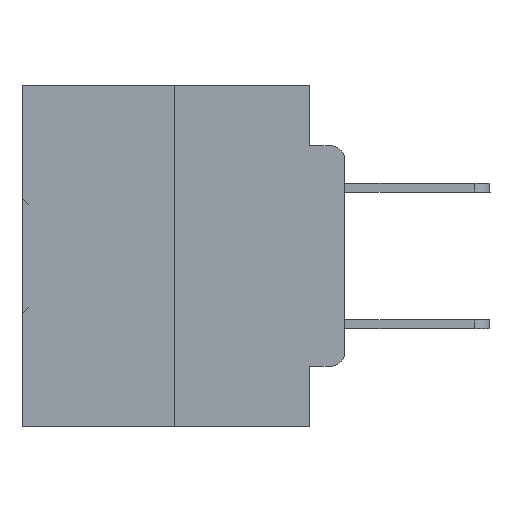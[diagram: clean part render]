
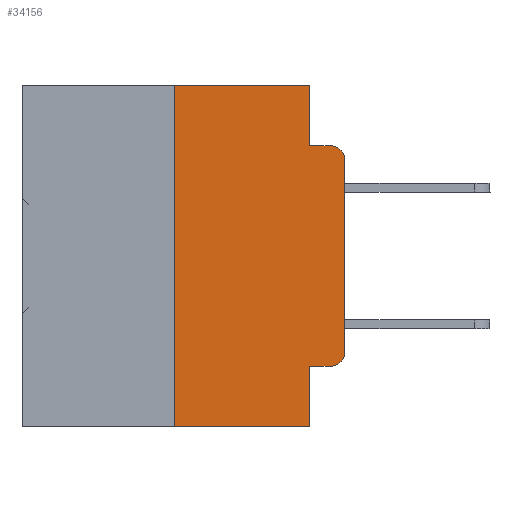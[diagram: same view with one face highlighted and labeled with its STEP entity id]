
A CAD part, left-side view. The second image highlights one B-rep face of the part: STEP entity #34156.
In plain terms, the highlighted planar face has unit normal (-1, 0, 0).
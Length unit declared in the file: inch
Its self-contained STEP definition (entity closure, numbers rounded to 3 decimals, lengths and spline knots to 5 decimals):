
#143 = VECTOR ( 'NONE', #10157, 39.37008 ) ;
#616 = ORIENTED_EDGE ( 'NONE', *, *, #23244, .F. ) ;
#656 = VERTEX_POINT ( 'NONE', #26328 ) ;
#908 = DIRECTION ( 'NONE',  ( -1., 0., 0. ) ) ;
#1549 = VERTEX_POINT ( 'NONE', #1915 ) ;
#1915 = CARTESIAN_POINT ( 'NONE',  ( 0., 0.051, -0.5 ) ) ;
#2710 = CARTESIAN_POINT ( 'NONE',  ( 0., 0.051, 0. ) ) ;
#4378 = EDGE_CURVE ( 'NONE', #37192, #1549, #31212, .T. ) ;
#4537 = VERTEX_POINT ( 'NONE', #11306 ) ;
#4974 = LINE ( 'NONE', #16615, #14057 ) ;
#5849 = CARTESIAN_POINT ( 'NONE',  ( 0., 0., 0. ) ) ;
#6620 = VECTOR ( 'NONE', #20495, 39.37008 ) ;
#6967 = EDGE_CURVE ( 'NONE', #656, #1549, #36945, .T. ) ;
#6978 = DIRECTION ( 'NONE',  ( 1., 0., 0. ) ) ;
#7118 = LINE ( 'NONE', #27726, #143 ) ;
#7808 = ORIENTED_EDGE ( 'NONE', *, *, #36953, .F. ) ;
#8787 = CARTESIAN_POINT ( 'NONE',  ( 0., 0.02, -0.0885 ) ) ;
#8930 = LINE ( 'NONE', #28993, #17694 ) ;
#9353 = AXIS2_PLACEMENT_3D ( 'NONE', #15770, #908, #24173 ) ;
#10157 = DIRECTION ( 'NONE',  ( 0., -1., 0. ) ) ;
#10760 = ORIENTED_EDGE ( 'NONE', *, *, #15031, .T. ) ;
#10908 = CARTESIAN_POINT ( 'NONE',  ( 0., 0., -0.3915 ) ) ;
#11306 = CARTESIAN_POINT ( 'NONE',  ( 0., 0.02, -0.4115 ) ) ;
#12842 = DIRECTION ( 'NONE',  ( 0., -1., 0. ) ) ;
#13607 = CARTESIAN_POINT ( 'NONE',  ( 0., 0.473, -0.5 ) ) ;
#14057 = VECTOR ( 'NONE', #24625, 39.37008 ) ;
#14627 = LINE ( 'NONE', #5849, #36885 ) ;
#15031 = EDGE_CURVE ( 'NONE', #4537, #23586, #25821, .T. ) ;
#15770 = CARTESIAN_POINT ( 'NONE',  ( 0., 0.02, -0.3915 ) ) ;
#15806 = VERTEX_POINT ( 'NONE', #17244 ) ;
#16136 = CIRCLE ( 'NONE', #21624, 0.02 ) ;
#16139 = ORIENTED_EDGE ( 'NONE', *, *, #6967, .F. ) ;
#16615 = CARTESIAN_POINT ( 'NONE',  ( 0., 0.051, 0. ) ) ;
#16894 = CARTESIAN_POINT ( 'NONE',  ( 0., 0.25, 0. ) ) ;
#16953 = EDGE_LOOP ( 'NONE', ( #18573, #20050, #22923, #31908, #7808, #616, #29682, #16139, #18388, #10760 ) ) ;
#17136 = DIRECTION ( 'NONE',  ( 0., 0., -1. ) ) ;
#17244 = CARTESIAN_POINT ( 'NONE',  ( 0., 0., -0.1085 ) ) ;
#17548 = VERTEX_POINT ( 'NONE', #8787 ) ;
#17694 = VECTOR ( 'NONE', #23618, 39.37008 ) ;
#18388 = ORIENTED_EDGE ( 'NONE', *, *, #27282, .T. ) ;
#18544 = VECTOR ( 'NONE', #12842, 39.37008 ) ;
#18573 = ORIENTED_EDGE ( 'NONE', *, *, #32778, .T. ) ;
#19003 = CARTESIAN_POINT ( 'NONE',  ( 0., 0.473, 0. ) ) ;
#19056 = VERTEX_POINT ( 'NONE', #36357 ) ;
#19998 = DIRECTION ( 'NONE',  ( -1., 0., 0. ) ) ;
#20050 = ORIENTED_EDGE ( 'NONE', *, *, #35152, .T. ) ;
#20133 = LINE ( 'NONE', #16894, #6620 ) ;
#20495 = DIRECTION ( 'NONE',  ( 0., 0., 1. ) ) ;
#20563 = VERTEX_POINT ( 'NONE', #22037 ) ;
#21624 = AXIS2_PLACEMENT_3D ( 'NONE', #34558, #19998, #17136 ) ;
#22037 = CARTESIAN_POINT ( 'NONE',  ( 0., 0.051, -0.0885 ) ) ;
#22040 = CARTESIAN_POINT ( 'NONE',  ( 0., 0.25, -0.5 ) ) ;
#22923 = ORIENTED_EDGE ( 'NONE', *, *, #30856, .F. ) ;
#22931 = DIRECTION ( 'NONE',  ( 0., 0., -1. ) ) ;
#23221 = VERTEX_POINT ( 'NONE', #34318 ) ;
#23244 = EDGE_CURVE ( 'NONE', #37192, #23221, #20133, .T. ) ;
#23586 = VERTEX_POINT ( 'NONE', #10908 ) ;
#23618 = DIRECTION ( 'NONE',  ( 0., -1., 0. ) ) ;
#24173 = DIRECTION ( 'NONE',  ( 0., 0., -1. ) ) ;
#24521 = PLANE ( 'NONE',  #33824 ) ;
#24625 = DIRECTION ( 'NONE',  ( 0., 0., -1. ) ) ;
#25346 = EDGE_CURVE ( 'NONE', #19056, #20563, #4974, .T. ) ;
#25392 = VECTOR ( 'NONE', #35849, 39.37008 ) ;
#25821 = CIRCLE ( 'NONE', #9353, 0.02 ) ;
#26328 = CARTESIAN_POINT ( 'NONE',  ( 0., 0.051, -0.4115 ) ) ;
#27282 = EDGE_CURVE ( 'NONE', #656, #4537, #8930, .T. ) ;
#27726 = CARTESIAN_POINT ( 'NONE',  ( 0., 0.051, -0.0885 ) ) ;
#28993 = CARTESIAN_POINT ( 'NONE',  ( 0., 0.051, -0.4115 ) ) ;
#29137 = DIRECTION ( 'NONE',  ( 0., 0., 1. ) ) ;
#29682 = ORIENTED_EDGE ( 'NONE', *, *, #4378, .T. ) ;
#30476 = FACE_OUTER_BOUND ( 'NONE', #16953, .T. ) ;
#30668 = DIRECTION ( 'NONE',  ( 0., 0., -1. ) ) ;
#30856 = EDGE_CURVE ( 'NONE', #20563, #17548, #7118, .T. ) ;
#31212 = LINE ( 'NONE', #13607, #18544 ) ;
#31908 = ORIENTED_EDGE ( 'NONE', *, *, #25346, .F. ) ;
#32778 = EDGE_CURVE ( 'NONE', #23586, #15806, #14627, .T. ) ;
#32782 = LINE ( 'NONE', #36417, #25392 ) ;
#33824 = AXIS2_PLACEMENT_3D ( 'NONE', #19003, #6978, #30668 ) ;
#34156 = ADVANCED_FACE ( 'NONE', ( #30476 ), #24521, .F. ) ;
#34318 = CARTESIAN_POINT ( 'NONE',  ( 0., 0.25, 0. ) ) ;
#34558 = CARTESIAN_POINT ( 'NONE',  ( 0., 0.02, -0.1085 ) ) ;
#35152 = EDGE_CURVE ( 'NONE', #15806, #17548, #16136, .T. ) ;
#35849 = DIRECTION ( 'NONE',  ( 0., -1., 0. ) ) ;
#36357 = CARTESIAN_POINT ( 'NONE',  ( 0., 0.051, 0. ) ) ;
#36417 = CARTESIAN_POINT ( 'NONE',  ( 0., 0.473, 0. ) ) ;
#36885 = VECTOR ( 'NONE', #29137, 39.37008 ) ;
#36945 = LINE ( 'NONE', #2710, #36988 ) ;
#36953 = EDGE_CURVE ( 'NONE', #23221, #19056, #32782, .T. ) ;
#36988 = VECTOR ( 'NONE', #22931, 39.37008 ) ;
#37192 = VERTEX_POINT ( 'NONE', #22040 ) ;
